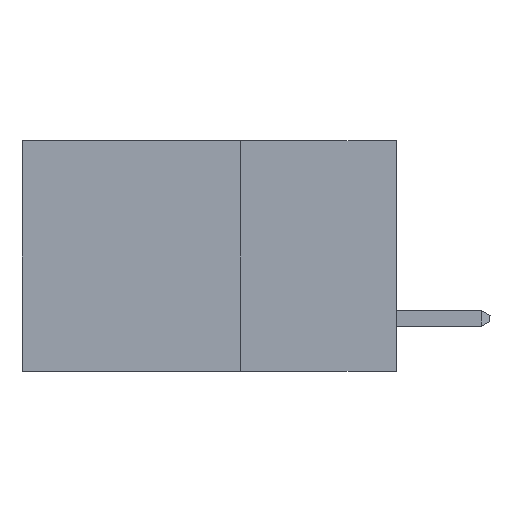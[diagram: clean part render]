
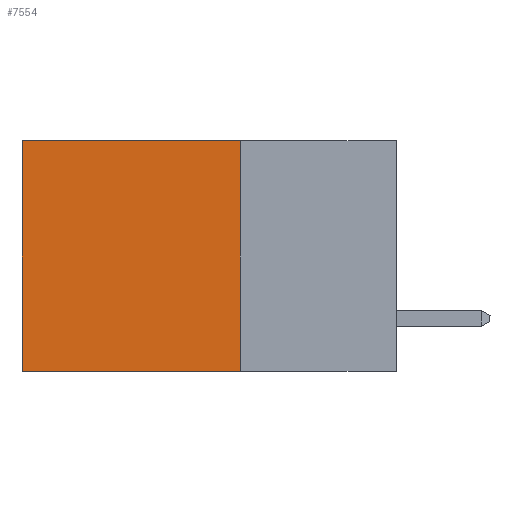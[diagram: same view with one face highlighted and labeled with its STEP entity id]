
A CAD part, left-side view. The second image highlights one B-rep face of the part: STEP entity #7554.
In plain terms, the highlighted planar face has unit normal (-1, 0, 0).
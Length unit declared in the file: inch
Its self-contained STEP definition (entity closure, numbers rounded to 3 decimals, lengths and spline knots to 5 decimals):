
#447 = LINE ( 'NONE', #2288, #2874 ) ;
#1126 = DIRECTION ( 'NONE',  ( 0., 0., -1. ) ) ;
#1769 = CARTESIAN_POINT ( 'NONE',  ( 0.2615, 0.25, -0.37 ) ) ;
#2288 = CARTESIAN_POINT ( 'NONE',  ( 0.2615, 0.6, -0.37 ) ) ;
#2425 = EDGE_CURVE ( 'NONE', #11476, #4382, #2935, .T. ) ;
#2609 = ORIENTED_EDGE ( 'NONE', *, *, #4438, .T. ) ;
#2874 = VECTOR ( 'NONE', #4147, 39.37008 ) ;
#2935 = LINE ( 'NONE', #9451, #8632 ) ;
#3833 = CARTESIAN_POINT ( 'NONE',  ( 0.2615, 0.25, 0. ) ) ;
#3887 = AXIS2_PLACEMENT_3D ( 'NONE', #8705, #6646, #3891 ) ;
#3891 = DIRECTION ( 'NONE',  ( 0., 0., -1. ) ) ;
#4147 = DIRECTION ( 'NONE',  ( 0., 0., -1. ) ) ;
#4304 = CARTESIAN_POINT ( 'NONE',  ( 0.2615, 0.6, -0.37 ) ) ;
#4382 = VERTEX_POINT ( 'NONE', #5526 ) ;
#4438 = EDGE_CURVE ( 'NONE', #11476, #5791, #5634, .T. ) ;
#4884 = DIRECTION ( 'NONE',  ( 0., 1., 0. ) ) ;
#5132 = ORIENTED_EDGE ( 'NONE', *, *, #2425, .F. ) ;
#5140 = LINE ( 'NONE', #1769, #11127 ) ;
#5405 = EDGE_CURVE ( 'NONE', #5791, #11552, #447, .T. ) ;
#5526 = CARTESIAN_POINT ( 'NONE',  ( 0.2615, 0.25, -0.37 ) ) ;
#5539 = CARTESIAN_POINT ( 'NONE',  ( 0.2615, 0.6, 0. ) ) ;
#5634 = LINE ( 'NONE', #3833, #10866 ) ;
#5791 = VERTEX_POINT ( 'NONE', #5539 ) ;
#6646 = DIRECTION ( 'NONE',  ( 1., 0., 0. ) ) ;
#7305 = EDGE_LOOP ( 'NONE', ( #8762, #11261, #5132, #2609 ) ) ;
#7554 = ADVANCED_FACE ( 'NONE', ( #10424 ), #10494, .F. ) ;
#7737 = CARTESIAN_POINT ( 'NONE',  ( 0.2615, 0.25, 0. ) ) ;
#8632 = VECTOR ( 'NONE', #1126, 39.37008 ) ;
#8705 = CARTESIAN_POINT ( 'NONE',  ( 0.2615, 0.25, -0.37 ) ) ;
#8762 = ORIENTED_EDGE ( 'NONE', *, *, #5405, .T. ) ;
#9049 = EDGE_CURVE ( 'NONE', #4382, #11552, #5140, .T. ) ;
#9451 = CARTESIAN_POINT ( 'NONE',  ( 0.2615, 0.25, -0.37 ) ) ;
#10424 = FACE_OUTER_BOUND ( 'NONE', #7305, .T. ) ;
#10494 = PLANE ( 'NONE',  #3887 ) ;
#10866 = VECTOR ( 'NONE', #4884, 39.37008 ) ;
#10977 = DIRECTION ( 'NONE',  ( 0., 1., 0. ) ) ;
#11127 = VECTOR ( 'NONE', #10977, 39.37008 ) ;
#11261 = ORIENTED_EDGE ( 'NONE', *, *, #9049, .F. ) ;
#11476 = VERTEX_POINT ( 'NONE', #7737 ) ;
#11552 = VERTEX_POINT ( 'NONE', #4304 ) ;
